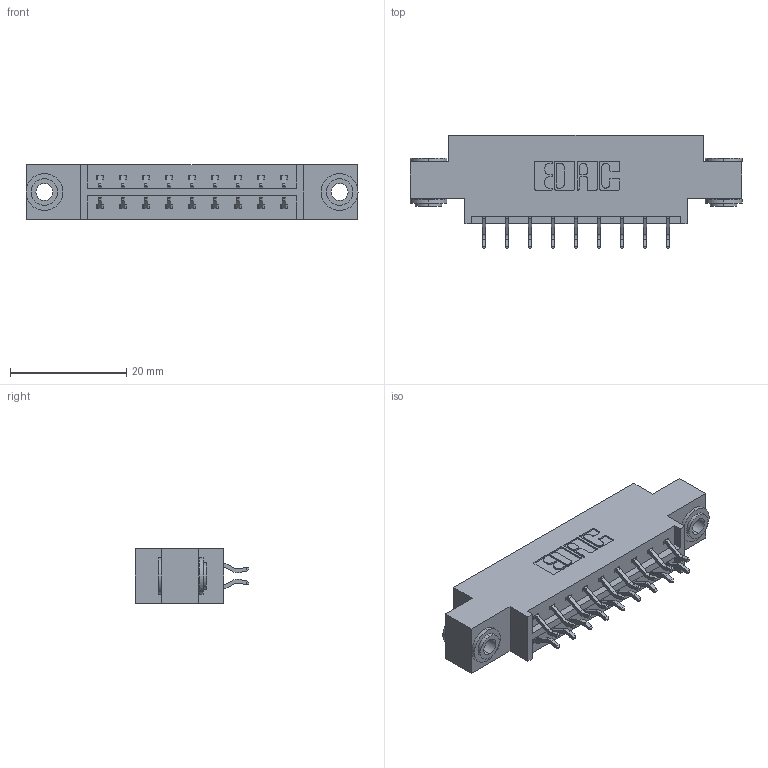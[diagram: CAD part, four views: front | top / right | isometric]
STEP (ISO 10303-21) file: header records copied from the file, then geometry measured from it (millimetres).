
FILE_DESCRIPTION (( 'STEP AP203' ), '1' );
FILE_NAME ('833-018-556-803.STEP', '2020-05-31T23:05:26', ( '' ), ( '' ), 'SwSTEP 2.0', 'SolidWorks 2020', '' );
FILE_SCHEMA (( 'CONFIG_CONTROL_DESIGN' ));
Length unit declared in the file: inch
Products named in the file (4): 345-250-002_345-250-002-102; 345-292-001_556 Tail; 833-018-556-803; 833 Part_Offset - .156 Dia - TH
Assembly tree (21 placements, depth 2):
  833-018-556-803
    833 Part_Offset - .156 Dia - TH
    345-292-001_556 Tail  x18
    345-250-002_345-250-002-102  x2
Bounding box: 57.2 x 19.57 x 9.4 mm (x, y, z)
Volume: 5322.2 mm3; surface area: 6361.5 mm2
Topology: 21 solids, 21 shells, 1200 faces, 3513 edges, 2314 vertices
Faces by surface type: plane 804, cylinder 388, cone 8
Entity records: 11060 total; most frequent: CARTESIAN_POINT 1865, ORIENTED_EDGE 1782, DIRECTION 1673, EDGE_CURVE 891, VECTOR 731, LINE 731, VERTEX_POINT 590, AXIS2_PLACEMENT_3D 471
